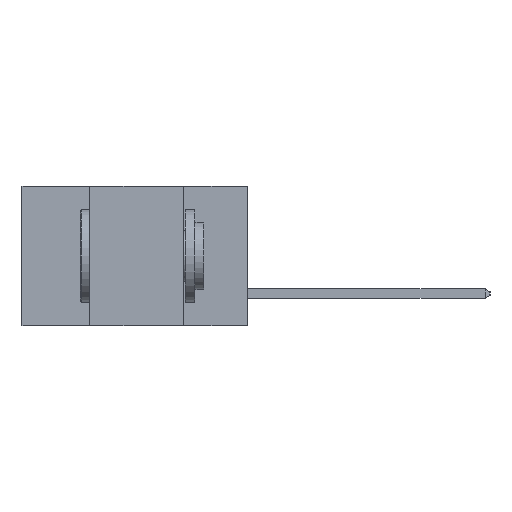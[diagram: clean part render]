
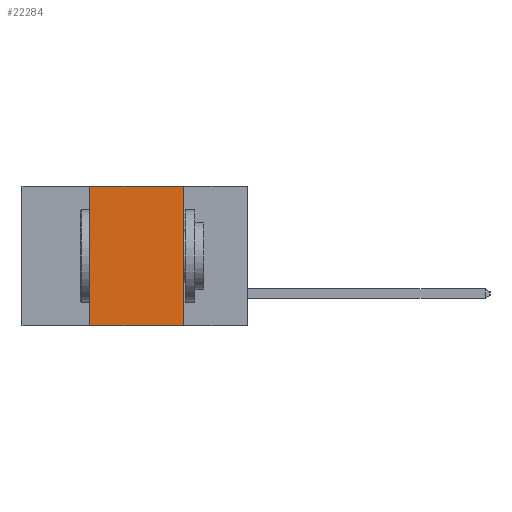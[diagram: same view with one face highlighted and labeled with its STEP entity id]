
A CAD part, left-side view. The second image highlights one B-rep face of the part: STEP entity #22284.
In plain terms, the highlighted planar face has unit normal (-1, 0, 0).
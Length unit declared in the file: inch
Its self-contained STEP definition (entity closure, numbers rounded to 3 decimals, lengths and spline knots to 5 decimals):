
#780 = CARTESIAN_POINT ( 'NONE',  ( 0., 0.42, -0.37 ) ) ;
#1042 = CARTESIAN_POINT ( 'NONE',  ( 0., 0.6, 0. ) ) ;
#1262 = VECTOR ( 'NONE', #15005, 39.37008 ) ;
#1313 = DIRECTION ( 'NONE',  ( 0., -1., 0. ) ) ;
#1727 = AXIS2_PLACEMENT_3D ( 'NONE', #1042, #13476, #2837 ) ;
#2306 = EDGE_CURVE ( 'NONE', #11920, #18079, #14904, .T. ) ;
#2728 = CARTESIAN_POINT ( 'NONE',  ( 0., 0.6, -0.37 ) ) ;
#2837 = DIRECTION ( 'NONE',  ( 0., 0., -1. ) ) ;
#5140 = VECTOR ( 'NONE', #13303, 39.37008 ) ;
#6086 = EDGE_LOOP ( 'NONE', ( #14606, #15718, #13776, #21140 ) ) ;
#9239 = CARTESIAN_POINT ( 'NONE',  ( 0., 0.17, -0.37 ) ) ;
#9671 = VECTOR ( 'NONE', #1313, 39.37008 ) ;
#10261 = VERTEX_POINT ( 'NONE', #18204 ) ;
#11920 = VERTEX_POINT ( 'NONE', #16904 ) ;
#12607 = LINE ( 'NONE', #19891, #21341 ) ;
#13303 = DIRECTION ( 'NONE',  ( 0., 0., 1. ) ) ;
#13476 = DIRECTION ( 'NONE',  ( 1., 0., 0. ) ) ;
#13776 = ORIENTED_EDGE ( 'NONE', *, *, #19415, .F. ) ;
#13899 = FACE_OUTER_BOUND ( 'NONE', #6086, .T. ) ;
#14399 = LINE ( 'NONE', #2728, #9671 ) ;
#14606 = ORIENTED_EDGE ( 'NONE', *, *, #2306, .F. ) ;
#14904 = LINE ( 'NONE', #19095, #1262 ) ;
#15005 = DIRECTION ( 'NONE',  ( 0., 0., -1. ) ) ;
#15021 = CARTESIAN_POINT ( 'NONE',  ( 0., 0.42, -0.37 ) ) ;
#15201 = LINE ( 'NONE', #15021, #5140 ) ;
#15718 = ORIENTED_EDGE ( 'NONE', *, *, #20517, .F. ) ;
#16342 = VERTEX_POINT ( 'NONE', #780 ) ;
#16904 = CARTESIAN_POINT ( 'NONE',  ( 0., 0.17, 0. ) ) ;
#17050 = EDGE_CURVE ( 'NONE', #16342, #18079, #14399, .T. ) ;
#18079 = VERTEX_POINT ( 'NONE', #9239 ) ;
#18204 = CARTESIAN_POINT ( 'NONE',  ( 0., 0.42, 0. ) ) ;
#18304 = DIRECTION ( 'NONE',  ( 0., -1., 0. ) ) ;
#18785 = PLANE ( 'NONE',  #1727 ) ;
#19095 = CARTESIAN_POINT ( 'NONE',  ( 0., 0.17, -0.37 ) ) ;
#19415 = EDGE_CURVE ( 'NONE', #16342, #10261, #15201, .T. ) ;
#19891 = CARTESIAN_POINT ( 'NONE',  ( 0., 0.6, 0. ) ) ;
#20517 = EDGE_CURVE ( 'NONE', #10261, #11920, #12607, .T. ) ;
#21140 = ORIENTED_EDGE ( 'NONE', *, *, #17050, .T. ) ;
#21341 = VECTOR ( 'NONE', #18304, 39.37008 ) ;
#22284 = ADVANCED_FACE ( 'NONE', ( #13899 ), #18785, .F. ) ;
